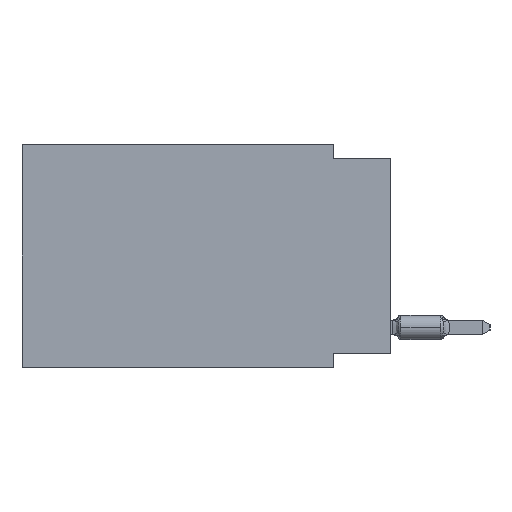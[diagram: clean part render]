
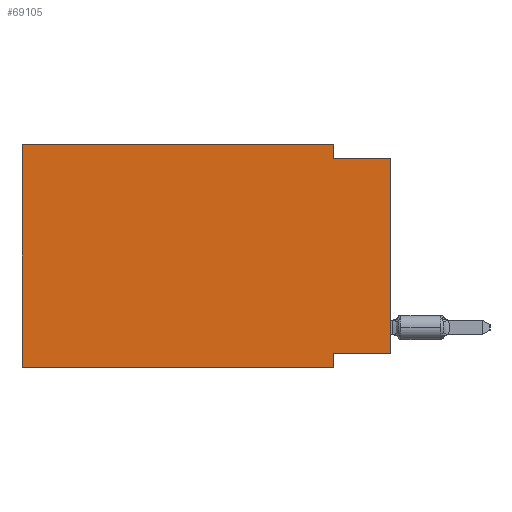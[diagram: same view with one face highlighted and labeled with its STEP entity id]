
A CAD part, left-side view. The second image highlights one B-rep face of the part: STEP entity #69105.
In plain terms, the highlighted planar face has unit normal (-1, 0, 0).
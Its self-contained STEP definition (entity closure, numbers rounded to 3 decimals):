
#1545 = VECTOR ( 'NONE', #57267, 1000. ) ;
#1820 = ORIENTED_EDGE ( 'NONE', *, *, #53551, .T. ) ;
#1846 = FACE_OUTER_BOUND ( 'NONE', #7542, .T. ) ;
#2190 = ORIENTED_EDGE ( 'NONE', *, *, #14704, .F. ) ;
#2829 = DIRECTION ( 'NONE',  ( 0., -1., 0. ) ) ;
#3602 = CARTESIAN_POINT ( 'NONE',  ( 0., 16.383, 0. ) ) ;
#4035 = EDGE_CURVE ( 'NONE', #36231, #49386, #72124, .T. ) ;
#4380 = VERTEX_POINT ( 'NONE', #61052 ) ;
#7302 = CARTESIAN_POINT ( 'NONE',  ( 0., 16.383, 0. ) ) ;
#7473 = EDGE_CURVE ( 'NONE', #66859, #76059, #56260, .T. ) ;
#7542 = EDGE_LOOP ( 'NONE', ( #49804, #63728, #36709, #12803, #44191, #1820, #16431, #2190 ) ) ;
#9849 = DIRECTION ( 'NONE',  ( 0., 0., 1. ) ) ;
#12803 = ORIENTED_EDGE ( 'NONE', *, *, #7473, .F. ) ;
#13057 = VECTOR ( 'NONE', #48675, 1000. ) ;
#14099 = LINE ( 'NONE', #74210, #71735 ) ;
#14139 = VERTEX_POINT ( 'NONE', #66413 ) ;
#14704 = EDGE_CURVE ( 'NONE', #36231, #56146, #34224, .T. ) ;
#16431 = ORIENTED_EDGE ( 'NONE', *, *, #73291, .F. ) ;
#18895 = EDGE_CURVE ( 'NONE', #76059, #28136, #14099, .T. ) ;
#19766 = LINE ( 'NONE', #37343, #27354 ) ;
#20200 = CARTESIAN_POINT ( 'NONE',  ( 0., 2.54, -0.635 ) ) ;
#25389 = CARTESIAN_POINT ( 'NONE',  ( 0., 0., -9.271 ) ) ;
#26460 = LINE ( 'NONE', #56516, #52259 ) ;
#26682 = CARTESIAN_POINT ( 'NONE',  ( 0., 2.54, -9.271 ) ) ;
#27029 = CARTESIAN_POINT ( 'NONE',  ( 0., 16.383, 0. ) ) ;
#27354 = VECTOR ( 'NONE', #49413, 1000. ) ;
#28136 = VERTEX_POINT ( 'NONE', #20200 ) ;
#33459 = CARTESIAN_POINT ( 'NONE',  ( 0., 0., -9.271 ) ) ;
#34224 = LINE ( 'NONE', #33459, #1545 ) ;
#34739 = VECTOR ( 'NONE', #2829, 1000. ) ;
#35060 = VECTOR ( 'NONE', #9849, 1000. ) ;
#36036 = LINE ( 'NONE', #48113, #59359 ) ;
#36231 = VERTEX_POINT ( 'NONE', #25389 ) ;
#36709 = ORIENTED_EDGE ( 'NONE', *, *, #18895, .F. ) ;
#36950 = PLANE ( 'NONE',  #76794 ) ;
#37343 = CARTESIAN_POINT ( 'NONE',  ( 0., 2.54, -9.906 ) ) ;
#37471 = CARTESIAN_POINT ( 'NONE',  ( 0., 2.54, 0. ) ) ;
#42441 = DIRECTION ( 'NONE',  ( 1., 0., 0. ) ) ;
#42723 = EDGE_CURVE ( 'NONE', #14139, #66859, #62173, .T. ) ;
#44191 = ORIENTED_EDGE ( 'NONE', *, *, #42723, .F. ) ;
#48113 = CARTESIAN_POINT ( 'NONE',  ( 0., 16.383, -9.906 ) ) ;
#48675 = DIRECTION ( 'NONE',  ( 0., 0., 1. ) ) ;
#49386 = VERTEX_POINT ( 'NONE', #73959 ) ;
#49413 = DIRECTION ( 'NONE',  ( 0., 0., -1. ) ) ;
#49508 = DIRECTION ( 'NONE',  ( 0., -1., 0. ) ) ;
#49804 = ORIENTED_EDGE ( 'NONE', *, *, #4035, .T. ) ;
#52259 = VECTOR ( 'NONE', #49508, 1000. ) ;
#53551 = EDGE_CURVE ( 'NONE', #14139, #4380, #36036, .T. ) ;
#56146 = VERTEX_POINT ( 'NONE', #26682 ) ;
#56260 = LINE ( 'NONE', #3602, #34739 ) ;
#56516 = CARTESIAN_POINT ( 'NONE',  ( 0., 0., -0.635 ) ) ;
#57267 = DIRECTION ( 'NONE',  ( 0., 1., 0. ) ) ;
#57438 = CARTESIAN_POINT ( 'NONE',  ( 0., 16.383, 0. ) ) ;
#59359 = VECTOR ( 'NONE', #59833, 1000. ) ;
#59833 = DIRECTION ( 'NONE',  ( 0., -1., 0. ) ) ;
#61052 = CARTESIAN_POINT ( 'NONE',  ( 0., 2.54, -9.906 ) ) ;
#62173 = LINE ( 'NONE', #57438, #35060 ) ;
#63728 = ORIENTED_EDGE ( 'NONE', *, *, #72945, .F. ) ;
#66413 = CARTESIAN_POINT ( 'NONE',  ( 0., 16.383, -9.906 ) ) ;
#66630 = DIRECTION ( 'NONE',  ( 0., 0., -1. ) ) ;
#66823 = DIRECTION ( 'NONE',  ( 0., 0., -1. ) ) ;
#66859 = VERTEX_POINT ( 'NONE', #27029 ) ;
#69105 = ADVANCED_FACE ( 'NONE', ( #1846 ), #36950, .F. ) ;
#71735 = VECTOR ( 'NONE', #66823, 1000. ) ;
#72124 = LINE ( 'NONE', #72890, #13057 ) ;
#72890 = CARTESIAN_POINT ( 'NONE',  ( 0., 0., 0. ) ) ;
#72945 = EDGE_CURVE ( 'NONE', #28136, #49386, #26460, .T. ) ;
#73291 = EDGE_CURVE ( 'NONE', #56146, #4380, #19766, .T. ) ;
#73959 = CARTESIAN_POINT ( 'NONE',  ( 0., 0., -0.635 ) ) ;
#74210 = CARTESIAN_POINT ( 'NONE',  ( 0., 2.54, 0. ) ) ;
#76059 = VERTEX_POINT ( 'NONE', #37471 ) ;
#76794 = AXIS2_PLACEMENT_3D ( 'NONE', #7302, #42441, #66630 ) ;
